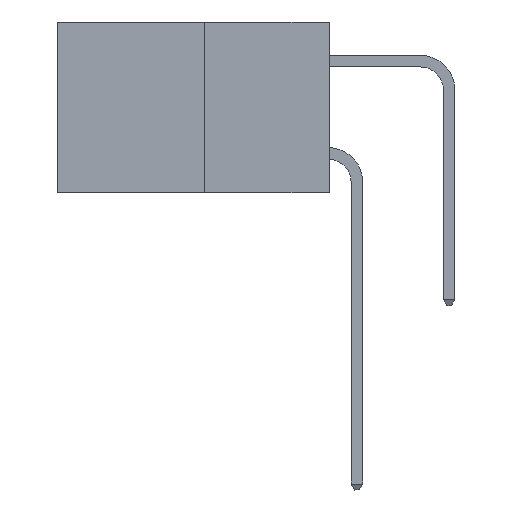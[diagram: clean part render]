
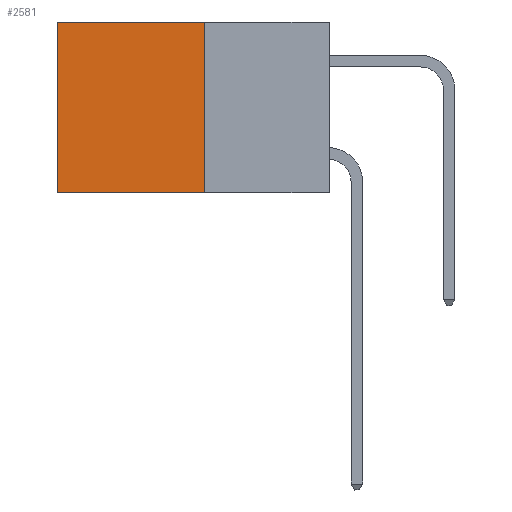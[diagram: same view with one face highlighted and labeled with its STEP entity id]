
A CAD part, left-side view. The second image highlights one B-rep face of the part: STEP entity #2581.
In plain terms, the highlighted planar face has unit normal (-1, 0, 0).
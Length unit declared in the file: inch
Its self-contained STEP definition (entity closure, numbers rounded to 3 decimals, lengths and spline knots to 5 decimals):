
#88 = VERTEX_POINT ( 'NONE', #8272 ) ;
#739 = DIRECTION ( 'NONE',  ( 1., 0., 0. ) ) ;
#775 = VECTOR ( 'NONE', #4044, 39.37008 ) ;
#949 = VECTOR ( 'NONE', #8813, 39.37008 ) ;
#1376 = CARTESIAN_POINT ( 'NONE',  ( 0.277, 0.27, -0.37 ) ) ;
#1561 = AXIS2_PLACEMENT_3D ( 'NONE', #7194, #739, #3102 ) ;
#1629 = EDGE_CURVE ( 'NONE', #2209, #88, #9629, .T. ) ;
#2169 = CARTESIAN_POINT ( 'NONE',  ( 0.277, 0.27, -0.37 ) ) ;
#2209 = VERTEX_POINT ( 'NONE', #10425 ) ;
#2572 = EDGE_LOOP ( 'NONE', ( #3627, #4396, #7067, #5041 ) ) ;
#2581 = ADVANCED_FACE ( 'NONE', ( #9906 ), #6414, .F. ) ;
#2765 = LINE ( 'NONE', #4841, #10116 ) ;
#3083 = EDGE_CURVE ( 'NONE', #8701, #6315, #6704, .T. ) ;
#3102 = DIRECTION ( 'NONE',  ( 0., 0., -1. ) ) ;
#3141 = DIRECTION ( 'NONE',  ( 0., 1., 0. ) ) ;
#3627 = ORIENTED_EDGE ( 'NONE', *, *, #3880, .T. ) ;
#3880 = EDGE_CURVE ( 'NONE', #6315, #88, #2765, .T. ) ;
#4044 = DIRECTION ( 'NONE',  ( 0., 1., 0. ) ) ;
#4396 = ORIENTED_EDGE ( 'NONE', *, *, #1629, .F. ) ;
#4557 = DIRECTION ( 'NONE',  ( 0., 0., -1. ) ) ;
#4841 = CARTESIAN_POINT ( 'NONE',  ( 0.277, 0.59, -0.37 ) ) ;
#5041 = ORIENTED_EDGE ( 'NONE', *, *, #3083, .T. ) ;
#5101 = EDGE_CURVE ( 'NONE', #8701, #2209, #6107, .T. ) ;
#6107 = LINE ( 'NONE', #2169, #949 ) ;
#6315 = VERTEX_POINT ( 'NONE', #10022 ) ;
#6414 = PLANE ( 'NONE',  #1561 ) ;
#6461 = VECTOR ( 'NONE', #3141, 39.37008 ) ;
#6704 = LINE ( 'NONE', #7190, #6461 ) ;
#7067 = ORIENTED_EDGE ( 'NONE', *, *, #5101, .F. ) ;
#7190 = CARTESIAN_POINT ( 'NONE',  ( 0.277, 0.27, 0. ) ) ;
#7194 = CARTESIAN_POINT ( 'NONE',  ( 0.277, 0.27, -0.37 ) ) ;
#8272 = CARTESIAN_POINT ( 'NONE',  ( 0.277, 0.59, -0.37 ) ) ;
#8701 = VERTEX_POINT ( 'NONE', #9585 ) ;
#8813 = DIRECTION ( 'NONE',  ( 0., 0., -1. ) ) ;
#9585 = CARTESIAN_POINT ( 'NONE',  ( 0.277, 0.27, 0. ) ) ;
#9629 = LINE ( 'NONE', #1376, #775 ) ;
#9906 = FACE_OUTER_BOUND ( 'NONE', #2572, .T. ) ;
#10022 = CARTESIAN_POINT ( 'NONE',  ( 0.277, 0.59, 0. ) ) ;
#10116 = VECTOR ( 'NONE', #4557, 39.37008 ) ;
#10425 = CARTESIAN_POINT ( 'NONE',  ( 0.277, 0.27, -0.37 ) ) ;
